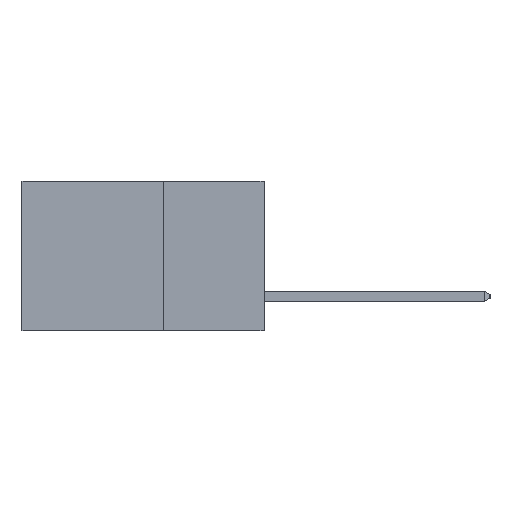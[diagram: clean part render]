
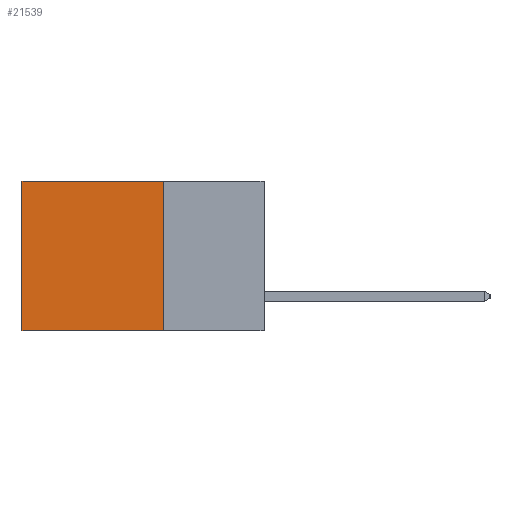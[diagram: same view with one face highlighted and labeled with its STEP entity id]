
A CAD part, left-side view. The second image highlights one B-rep face of the part: STEP entity #21539.
In plain terms, the highlighted planar face has unit normal (-1, 0, 0).
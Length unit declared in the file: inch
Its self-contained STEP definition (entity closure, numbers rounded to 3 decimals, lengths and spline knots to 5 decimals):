
#713 = AXIS2_PLACEMENT_3D ( 'NONE', #8192, #9927, #21722 ) ;
#3040 = EDGE_CURVE ( 'NONE', #17321, #10425, #20936, .T. ) ;
#3498 = LINE ( 'NONE', #8754, #7039 ) ;
#4579 = VERTEX_POINT ( 'NONE', #4857 ) ;
#4857 = CARTESIAN_POINT ( 'NONE',  ( 0.2615, 0.6, -0.37 ) ) ;
#4925 = ORIENTED_EDGE ( 'NONE', *, *, #3040, .F. ) ;
#6129 = EDGE_CURVE ( 'NONE', #10425, #4579, #3498, .T. ) ;
#6843 = VECTOR ( 'NONE', #15462, 39.37008 ) ;
#6892 = ORIENTED_EDGE ( 'NONE', *, *, #6129, .F. ) ;
#7039 = VECTOR ( 'NONE', #8114, 39.37008 ) ;
#7110 = CARTESIAN_POINT ( 'NONE',  ( 0.2615, 0.6, 0. ) ) ;
#7554 = VERTEX_POINT ( 'NONE', #7110 ) ;
#7821 = FACE_OUTER_BOUND ( 'NONE', #13385, .T. ) ;
#8114 = DIRECTION ( 'NONE',  ( 0., 1., 0. ) ) ;
#8192 = CARTESIAN_POINT ( 'NONE',  ( 0.2615, 0.25, -0.37 ) ) ;
#8335 = LINE ( 'NONE', #10973, #8902 ) ;
#8754 = CARTESIAN_POINT ( 'NONE',  ( 0.2615, 0.25, -0.37 ) ) ;
#8902 = VECTOR ( 'NONE', #17743, 39.37008 ) ;
#9927 = DIRECTION ( 'NONE',  ( 1., 0., 0. ) ) ;
#10425 = VERTEX_POINT ( 'NONE', #17653 ) ;
#10973 = CARTESIAN_POINT ( 'NONE',  ( 0.2615, 0.25, 0. ) ) ;
#12542 = EDGE_CURVE ( 'NONE', #7554, #4579, #19330, .T. ) ;
#13385 = EDGE_LOOP ( 'NONE', ( #16420, #6892, #4925, #14177 ) ) ;
#14177 = ORIENTED_EDGE ( 'NONE', *, *, #21933, .T. ) ;
#14815 = VECTOR ( 'NONE', #20069, 39.37008 ) ;
#15462 = DIRECTION ( 'NONE',  ( 0., 0., -1. ) ) ;
#16152 = CARTESIAN_POINT ( 'NONE',  ( 0.2615, 0.25, -0.37 ) ) ;
#16420 = ORIENTED_EDGE ( 'NONE', *, *, #12542, .T. ) ;
#17321 = VERTEX_POINT ( 'NONE', #19141 ) ;
#17653 = CARTESIAN_POINT ( 'NONE',  ( 0.2615, 0.25, -0.37 ) ) ;
#17743 = DIRECTION ( 'NONE',  ( 0., 1., 0. ) ) ;
#18411 = PLANE ( 'NONE',  #713 ) ;
#19141 = CARTESIAN_POINT ( 'NONE',  ( 0.2615, 0.25, 0. ) ) ;
#19330 = LINE ( 'NONE', #20202, #14815 ) ;
#20069 = DIRECTION ( 'NONE',  ( 0., 0., -1. ) ) ;
#20202 = CARTESIAN_POINT ( 'NONE',  ( 0.2615, 0.6, -0.37 ) ) ;
#20936 = LINE ( 'NONE', #16152, #6843 ) ;
#21539 = ADVANCED_FACE ( 'NONE', ( #7821 ), #18411, .F. ) ;
#21722 = DIRECTION ( 'NONE',  ( 0., 0., -1. ) ) ;
#21933 = EDGE_CURVE ( 'NONE', #17321, #7554, #8335, .T. ) ;
